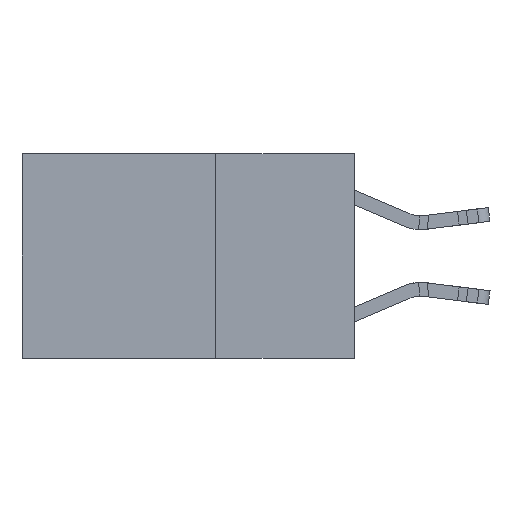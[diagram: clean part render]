
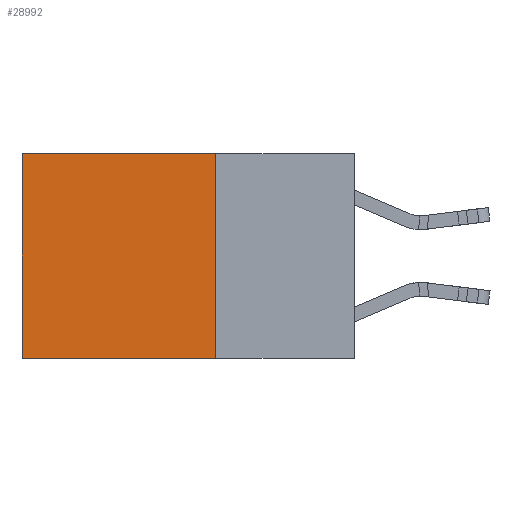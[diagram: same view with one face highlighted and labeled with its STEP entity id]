
A CAD part, left-side view. The second image highlights one B-rep face of the part: STEP entity #28992.
In plain terms, the highlighted planar face has unit normal (-1, 0, 0).
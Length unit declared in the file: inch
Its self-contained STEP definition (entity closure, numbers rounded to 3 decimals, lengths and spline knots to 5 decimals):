
#488 = CARTESIAN_POINT ( 'NONE',  ( 0.2625, 0.25, -0.37 ) ) ;
#1411 = EDGE_CURVE ( 'NONE', #21661, #1556, #2162, .T. ) ;
#1444 = DIRECTION ( 'NONE',  ( 1., 0., 0. ) ) ;
#1556 = VERTEX_POINT ( 'NONE', #4711 ) ;
#1748 = ORIENTED_EDGE ( 'NONE', *, *, #26405, .T. ) ;
#1794 = AXIS2_PLACEMENT_3D ( 'NONE', #28094, #1444, #17373 ) ;
#2162 = LINE ( 'NONE', #15624, #8228 ) ;
#4711 = CARTESIAN_POINT ( 'NONE',  ( 0.2625, 0.25, -0.37 ) ) ;
#4814 = VECTOR ( 'NONE', #18699, 39.37008 ) ;
#5856 = LINE ( 'NONE', #28456, #17231 ) ;
#7415 = ORIENTED_EDGE ( 'NONE', *, *, #1411, .F. ) ;
#8195 = DIRECTION ( 'NONE',  ( 0., 0., -1. ) ) ;
#8228 = VECTOR ( 'NONE', #29126, 39.37008 ) ;
#10009 = PLANE ( 'NONE',  #1794 ) ;
#11036 = ORIENTED_EDGE ( 'NONE', *, *, #15901, .F. ) ;
#12928 = DIRECTION ( 'NONE',  ( 0., 1., 0. ) ) ;
#15105 = CARTESIAN_POINT ( 'NONE',  ( 0.2625, 0.25, 0. ) ) ;
#15624 = CARTESIAN_POINT ( 'NONE',  ( 0.2625, 0.25, 0. ) ) ;
#15901 = EDGE_CURVE ( 'NONE', #1556, #26088, #28862, .T. ) ;
#17049 = CARTESIAN_POINT ( 'NONE',  ( 0.2625, 0.6, 0. ) ) ;
#17231 = VECTOR ( 'NONE', #8195, 39.37008 ) ;
#17373 = DIRECTION ( 'NONE',  ( 0., 0., -1. ) ) ;
#18699 = DIRECTION ( 'NONE',  ( 0., 1., 0. ) ) ;
#20166 = ORIENTED_EDGE ( 'NONE', *, *, #21116, .T. ) ;
#20522 = VERTEX_POINT ( 'NONE', #17049 ) ;
#20637 = VECTOR ( 'NONE', #12928, 39.37008 ) ;
#21116 = EDGE_CURVE ( 'NONE', #20522, #26088, #5856, .T. ) ;
#21661 = VERTEX_POINT ( 'NONE', #23528 ) ;
#22543 = EDGE_LOOP ( 'NONE', ( #20166, #11036, #7415, #1748 ) ) ;
#23528 = CARTESIAN_POINT ( 'NONE',  ( 0.2625, 0.25, 0. ) ) ;
#23972 = FACE_OUTER_BOUND ( 'NONE', #22543, .T. ) ;
#24567 = CARTESIAN_POINT ( 'NONE',  ( 0.2625, 0.6, -0.37 ) ) ;
#26088 = VERTEX_POINT ( 'NONE', #24567 ) ;
#26405 = EDGE_CURVE ( 'NONE', #21661, #20522, #26623, .T. ) ;
#26623 = LINE ( 'NONE', #15105, #20637 ) ;
#28094 = CARTESIAN_POINT ( 'NONE',  ( 0.2625, 0.25, 0. ) ) ;
#28456 = CARTESIAN_POINT ( 'NONE',  ( 0.2625, 0.6, 0. ) ) ;
#28862 = LINE ( 'NONE', #488, #4814 ) ;
#28992 = ADVANCED_FACE ( 'NONE', ( #23972 ), #10009, .F. ) ;
#29126 = DIRECTION ( 'NONE',  ( 0., 0., -1. ) ) ;
